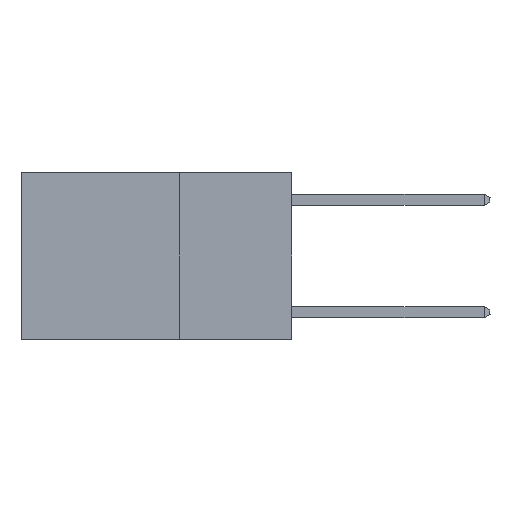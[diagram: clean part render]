
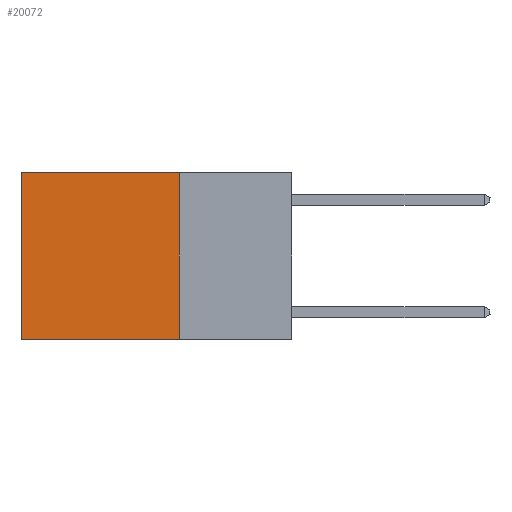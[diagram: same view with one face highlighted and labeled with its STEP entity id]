
A CAD part, left-side view. The second image highlights one B-rep face of the part: STEP entity #20072.
In plain terms, the highlighted planar face has unit normal (-1, 0, 0).
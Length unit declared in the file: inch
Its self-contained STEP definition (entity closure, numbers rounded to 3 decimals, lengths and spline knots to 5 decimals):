
#1415 = DIRECTION ( 'NONE',  ( 1., 0., 0. ) ) ;
#1649 = PLANE ( 'NONE',  #5372 ) ;
#2041 = CARTESIAN_POINT ( 'NONE',  ( 0.2625, 0.6, 0. ) ) ;
#2146 = VECTOR ( 'NONE', #11758, 39.37008 ) ;
#2433 = CARTESIAN_POINT ( 'NONE',  ( 0.2625, 0.6, 0. ) ) ;
#3023 = CARTESIAN_POINT ( 'NONE',  ( 0.2625, 0.25, 0. ) ) ;
#3194 = DIRECTION ( 'NONE',  ( 0., 0., -1. ) ) ;
#4108 = CARTESIAN_POINT ( 'NONE',  ( 0.2625, 0.25, 0. ) ) ;
#4419 = ORIENTED_EDGE ( 'NONE', *, *, #16185, .F. ) ;
#4738 = FACE_OUTER_BOUND ( 'NONE', #12466, .T. ) ;
#5010 = VERTEX_POINT ( 'NONE', #10391 ) ;
#5372 = AXIS2_PLACEMENT_3D ( 'NONE', #3023, #1415, #13553 ) ;
#6058 = DIRECTION ( 'NONE',  ( 0., 1., 0. ) ) ;
#6516 = VECTOR ( 'NONE', #6058, 39.37008 ) ;
#7768 = LINE ( 'NONE', #14642, #6516 ) ;
#7967 = LINE ( 'NONE', #13662, #2146 ) ;
#9131 = ORIENTED_EDGE ( 'NONE', *, *, #21626, .T. ) ;
#9265 = VERTEX_POINT ( 'NONE', #9523 ) ;
#9523 = CARTESIAN_POINT ( 'NONE',  ( 0.2625, 0.6, -0.37 ) ) ;
#10391 = CARTESIAN_POINT ( 'NONE',  ( 0.2625, 0.25, -0.37 ) ) ;
#11301 = DIRECTION ( 'NONE',  ( 0., 0., -1. ) ) ;
#11758 = DIRECTION ( 'NONE',  ( 0., 1., 0. ) ) ;
#12466 = EDGE_LOOP ( 'NONE', ( #9131, #4419, #18162, #15162 ) ) ;
#13500 = LINE ( 'NONE', #18627, #15620 ) ;
#13553 = DIRECTION ( 'NONE',  ( 0., 0., -1. ) ) ;
#13637 = VECTOR ( 'NONE', #11301, 39.37008 ) ;
#13662 = CARTESIAN_POINT ( 'NONE',  ( 0.2625, 0.25, -0.37 ) ) ;
#13880 = VERTEX_POINT ( 'NONE', #4108 ) ;
#14642 = CARTESIAN_POINT ( 'NONE',  ( 0.2625, 0.25, 0. ) ) ;
#15162 = ORIENTED_EDGE ( 'NONE', *, *, #15774, .T. ) ;
#15620 = VECTOR ( 'NONE', #3194, 39.37008 ) ;
#15774 = EDGE_CURVE ( 'NONE', #13880, #22326, #7768, .T. ) ;
#16185 = EDGE_CURVE ( 'NONE', #5010, #9265, #7967, .T. ) ;
#18162 = ORIENTED_EDGE ( 'NONE', *, *, #22213, .F. ) ;
#18627 = CARTESIAN_POINT ( 'NONE',  ( 0.2625, 0.25, 0. ) ) ;
#20072 = ADVANCED_FACE ( 'NONE', ( #4738 ), #1649, .F. ) ;
#21626 = EDGE_CURVE ( 'NONE', #22326, #9265, #21831, .T. ) ;
#21831 = LINE ( 'NONE', #2433, #13637 ) ;
#22213 = EDGE_CURVE ( 'NONE', #13880, #5010, #13500, .T. ) ;
#22326 = VERTEX_POINT ( 'NONE', #2041 ) ;
